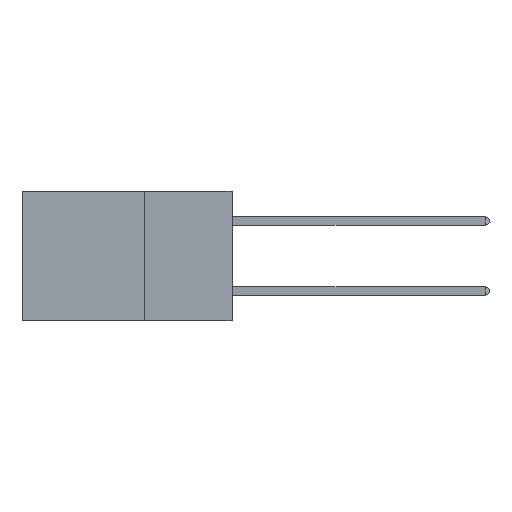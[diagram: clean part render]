
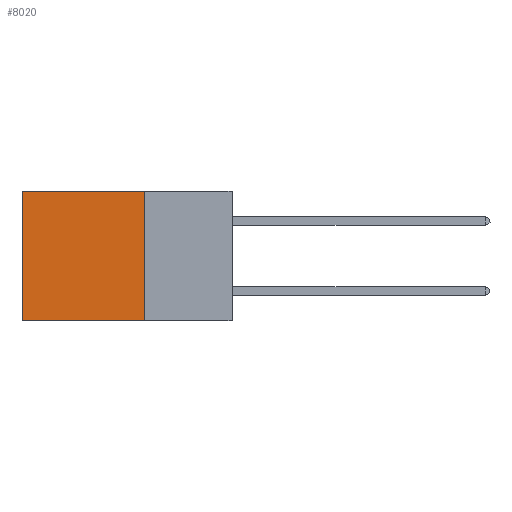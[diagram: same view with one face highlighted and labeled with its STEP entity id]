
A CAD part, left-side view. The second image highlights one B-rep face of the part: STEP entity #8020.
In plain terms, the highlighted planar face has unit normal (-1, 0, 0).
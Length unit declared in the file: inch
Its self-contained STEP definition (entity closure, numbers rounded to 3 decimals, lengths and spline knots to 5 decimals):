
#4324 = CARTESIAN_POINT ( 'NONE',  ( 0.2875, 0.25, 0. ) ) ;
#5530 = ORIENTED_EDGE ( 'NONE', *, *, #6132, .F. ) ;
#5662 = ORIENTED_EDGE ( 'NONE', *, *, #20582, .T. ) ;
#6132 = EDGE_CURVE ( 'NONE', #18340, #31492, #29301, .T. ) ;
#6308 = VECTOR ( 'NONE', #36801, 39.37008 ) ;
#8020 = ADVANCED_FACE ( 'NONE', ( #27153 ), #14142, .F. ) ;
#8508 = EDGE_LOOP ( 'NONE', ( #5662, #37285, #5530, #22174 ) ) ;
#10612 = EDGE_CURVE ( 'NONE', #18340, #25802, #15856, .T. ) ;
#11033 = DIRECTION ( 'NONE',  ( 0., 0., -1. ) ) ;
#12819 = VECTOR ( 'NONE', #29346, 39.37008 ) ;
#13463 = AXIS2_PLACEMENT_3D ( 'NONE', #26838, #14559, #11033 ) ;
#14142 = PLANE ( 'NONE',  #13463 ) ;
#14559 = DIRECTION ( 'NONE',  ( 1., 0., 0. ) ) ;
#15434 = CARTESIAN_POINT ( 'NONE',  ( 0.2875, 0.6, -0.37 ) ) ;
#15856 = LINE ( 'NONE', #4324, #40038 ) ;
#16138 = EDGE_CURVE ( 'NONE', #31492, #26220, #19991, .T. ) ;
#18340 = VERTEX_POINT ( 'NONE', #34320 ) ;
#19991 = LINE ( 'NONE', #37206, #6308 ) ;
#20582 = EDGE_CURVE ( 'NONE', #25802, #26220, #22426, .T. ) ;
#20759 = VECTOR ( 'NONE', #35534, 39.37008 ) ;
#22174 = ORIENTED_EDGE ( 'NONE', *, *, #10612, .T. ) ;
#22426 = LINE ( 'NONE', #26119, #12819 ) ;
#25802 = VERTEX_POINT ( 'NONE', #35584 ) ;
#26119 = CARTESIAN_POINT ( 'NONE',  ( 0.2875, 0.6, 0. ) ) ;
#26220 = VERTEX_POINT ( 'NONE', #15434 ) ;
#26838 = CARTESIAN_POINT ( 'NONE',  ( 0.2875, 0.25, 0. ) ) ;
#26938 = DIRECTION ( 'NONE',  ( 0., 1., 0. ) ) ;
#27153 = FACE_OUTER_BOUND ( 'NONE', #8508, .T. ) ;
#29301 = LINE ( 'NONE', #38777, #20759 ) ;
#29346 = DIRECTION ( 'NONE',  ( 0., 0., -1. ) ) ;
#31492 = VERTEX_POINT ( 'NONE', #39314 ) ;
#34320 = CARTESIAN_POINT ( 'NONE',  ( 0.2875, 0.25, 0. ) ) ;
#35534 = DIRECTION ( 'NONE',  ( 0., 0., -1. ) ) ;
#35584 = CARTESIAN_POINT ( 'NONE',  ( 0.2875, 0.6, 0. ) ) ;
#36801 = DIRECTION ( 'NONE',  ( 0., 1., 0. ) ) ;
#37206 = CARTESIAN_POINT ( 'NONE',  ( 0.2875, 0.25, -0.37 ) ) ;
#37285 = ORIENTED_EDGE ( 'NONE', *, *, #16138, .F. ) ;
#38777 = CARTESIAN_POINT ( 'NONE',  ( 0.2875, 0.25, 0. ) ) ;
#39314 = CARTESIAN_POINT ( 'NONE',  ( 0.2875, 0.25, -0.37 ) ) ;
#40038 = VECTOR ( 'NONE', #26938, 39.37008 ) ;
